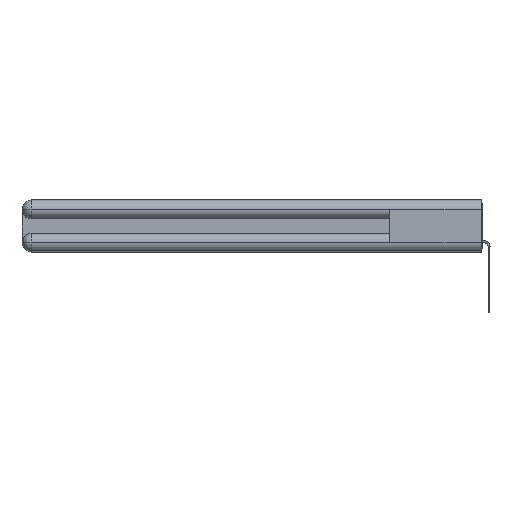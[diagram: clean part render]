
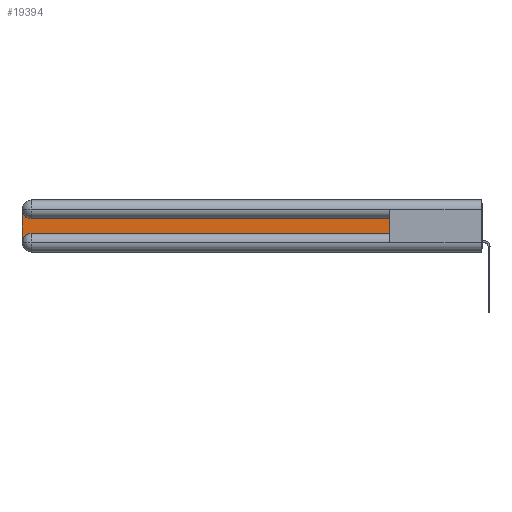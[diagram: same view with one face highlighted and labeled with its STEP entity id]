
A CAD part, left-side view. The second image highlights one B-rep face of the part: STEP entity #19394.
In plain terms, the highlighted planar face has unit normal (-1, 0, 0).
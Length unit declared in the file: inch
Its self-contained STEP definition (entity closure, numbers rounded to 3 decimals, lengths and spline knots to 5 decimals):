
#22 = AXIS2_PLACEMENT_3D ( 'NONE', #9792, #7274, #9520 ) ;
#38 = ORIENTED_EDGE ( 'NONE', *, *, #15201, .T. ) ;
#792 = VERTEX_POINT ( 'NONE', #20179 ) ;
#889 = VERTEX_POINT ( 'NONE', #3181 ) ;
#1119 = ORIENTED_EDGE ( 'NONE', *, *, #23150, .T. ) ;
#1839 = EDGE_CURVE ( 'NONE', #4908, #9565, #10225, .T. ) ;
#2099 = LINE ( 'NONE', #27223, #26788 ) ;
#3181 = CARTESIAN_POINT ( 'NONE',  ( 0.075, 3., -0.2775 ) ) ;
#3202 = ORIENTED_EDGE ( 'NONE', *, *, #1839, .T. ) ;
#3997 = EDGE_LOOP ( 'NONE', ( #19158, #13788, #1119, #19574, #38, #3202 ) ) ;
#4708 = EDGE_CURVE ( 'NONE', #792, #15706, #8050, .T. ) ;
#4908 = VERTEX_POINT ( 'NONE', #11555 ) ;
#6618 = CARTESIAN_POINT ( 'NONE',  ( 0.075, 0.6, -0.1225 ) ) ;
#7274 = DIRECTION ( 'NONE',  ( 1., 0., 0. ) ) ;
#7928 = DIRECTION ( 'NONE',  ( 1., 0., 0. ) ) ;
#8050 = CIRCLE ( 'NONE', #17497, 0.06 ) ;
#8277 = CARTESIAN_POINT ( 'NONE',  ( 0.075, 3., -0.2175 ) ) ;
#9105 = PLANE ( 'NONE',  #22 ) ;
#9520 = DIRECTION ( 'NONE',  ( 0., 0., -1. ) ) ;
#9565 = VERTEX_POINT ( 'NONE', #10795 ) ;
#9792 = CARTESIAN_POINT ( 'NONE',  ( 0.075, 3., -0.1225 ) ) ;
#10225 = LINE ( 'NONE', #14599, #19420 ) ;
#10330 = CARTESIAN_POINT ( 'NONE',  ( 0.075, 2.94, -0.2775 ) ) ;
#10655 = DIRECTION ( 'NONE',  ( 0., -1., 0. ) ) ;
#10755 = DIRECTION ( 'NONE',  ( 1., 0., 0. ) ) ;
#10795 = CARTESIAN_POINT ( 'NONE',  ( 0.075, 0.6, -0.1225 ) ) ;
#10977 = VECTOR ( 'NONE', #27502, 39.37008 ) ;
#11555 = CARTESIAN_POINT ( 'NONE',  ( 0.075, 0.6, -0.2175 ) ) ;
#12333 = DIRECTION ( 'NONE',  ( 0., 0., 1. ) ) ;
#12554 = CARTESIAN_POINT ( 'NONE',  ( 0.075, 3., -0.0625 ) ) ;
#13479 = LINE ( 'NONE', #6618, #21652 ) ;
#13652 = EDGE_CURVE ( 'NONE', #9565, #792, #13479, .T. ) ;
#13788 = ORIENTED_EDGE ( 'NONE', *, *, #4708, .T. ) ;
#14599 = CARTESIAN_POINT ( 'NONE',  ( 0.075, 0.6, -0.2175 ) ) ;
#15201 = EDGE_CURVE ( 'NONE', #22782, #4908, #2099, .T. ) ;
#15706 = VERTEX_POINT ( 'NONE', #12554 ) ;
#16898 = CARTESIAN_POINT ( 'NONE',  ( 0.075, 2.94, -0.2175 ) ) ;
#16940 = DIRECTION ( 'NONE',  ( 0., 0., -1. ) ) ;
#17497 = AXIS2_PLACEMENT_3D ( 'NONE', #25337, #7928, #16940 ) ;
#19158 = ORIENTED_EDGE ( 'NONE', *, *, #13652, .T. ) ;
#19394 = ADVANCED_FACE ( 'NONE', ( #19785 ), #9105, .F. ) ;
#19420 = VECTOR ( 'NONE', #12333, 39.37008 ) ;
#19574 = ORIENTED_EDGE ( 'NONE', *, *, #20661, .T. ) ;
#19785 = FACE_OUTER_BOUND ( 'NONE', #3997, .T. ) ;
#20179 = CARTESIAN_POINT ( 'NONE',  ( 0.075, 2.94, -0.1225 ) ) ;
#20661 = EDGE_CURVE ( 'NONE', #889, #22782, #23460, .T. ) ;
#21652 = VECTOR ( 'NONE', #23735, 39.37008 ) ;
#22782 = VERTEX_POINT ( 'NONE', #16898 ) ;
#22970 = DIRECTION ( 'NONE',  ( 0., 0., -1. ) ) ;
#23150 = EDGE_CURVE ( 'NONE', #15706, #889, #25410, .T. ) ;
#23460 = CIRCLE ( 'NONE', #24796, 0.06 ) ;
#23735 = DIRECTION ( 'NONE',  ( 0., 1., 0. ) ) ;
#24796 = AXIS2_PLACEMENT_3D ( 'NONE', #10330, #10755, #22970 ) ;
#25337 = CARTESIAN_POINT ( 'NONE',  ( 0.075, 2.94, -0.0625 ) ) ;
#25410 = LINE ( 'NONE', #8277, #10977 ) ;
#26788 = VECTOR ( 'NONE', #10655, 39.37008 ) ;
#27223 = CARTESIAN_POINT ( 'NONE',  ( 0.075, 0.6, -0.2175 ) ) ;
#27502 = DIRECTION ( 'NONE',  ( 0., 0., -1. ) ) ;
